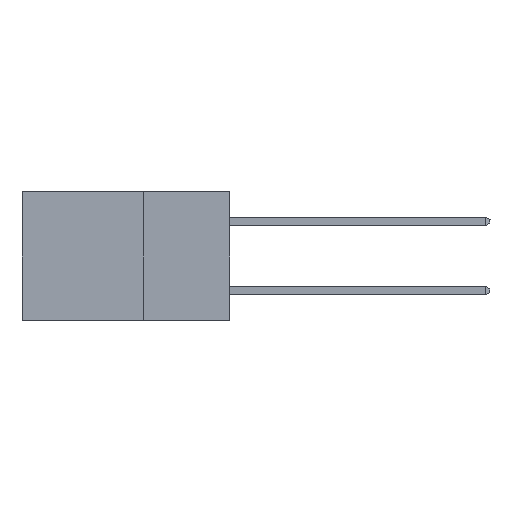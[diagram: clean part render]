
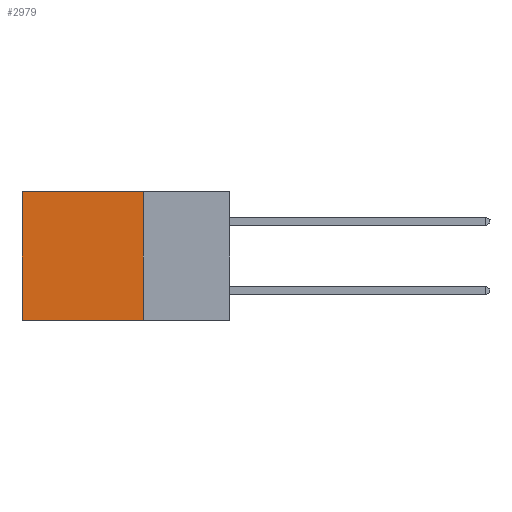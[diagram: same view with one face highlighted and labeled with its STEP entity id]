
A CAD part, left-side view. The second image highlights one B-rep face of the part: STEP entity #2979.
In plain terms, the highlighted planar face has unit normal (-1, 0, 0).
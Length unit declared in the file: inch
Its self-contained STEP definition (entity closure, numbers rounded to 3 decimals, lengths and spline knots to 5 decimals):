
#1040 = DIRECTION ( 'NONE',  ( 1., 0., 0. ) ) ;
#2979 = ADVANCED_FACE ( 'NONE', ( #11093 ), #12424, .F. ) ;
#3132 = AXIS2_PLACEMENT_3D ( 'NONE', #5033, #1040, #6096 ) ;
#3693 = EDGE_CURVE ( 'NONE', #15680, #8187, #13359, .T. ) ;
#4676 = VECTOR ( 'NONE', #14697, 39.37008 ) ;
#4803 = DIRECTION ( 'NONE',  ( 0., 1., 0. ) ) ;
#5033 = CARTESIAN_POINT ( 'NONE',  ( 0.2615, 0.25, -0.37 ) ) ;
#5502 = VECTOR ( 'NONE', #9378, 39.37008 ) ;
#5629 = CARTESIAN_POINT ( 'NONE',  ( 0.2615, 0.25, -0.37 ) ) ;
#6096 = DIRECTION ( 'NONE',  ( 0., 0., -1. ) ) ;
#6901 = EDGE_CURVE ( 'NONE', #7925, #8187, #10790, .T. ) ;
#7024 = CARTESIAN_POINT ( 'NONE',  ( 0.2615, 0.25, -0.37 ) ) ;
#7925 = VERTEX_POINT ( 'NONE', #5629 ) ;
#8187 = VERTEX_POINT ( 'NONE', #14788 ) ;
#9378 = DIRECTION ( 'NONE',  ( 0., 0., -1. ) ) ;
#9554 = LINE ( 'NONE', #15711, #5502 ) ;
#9958 = CARTESIAN_POINT ( 'NONE',  ( 0.2615, 0.25, 0. ) ) ;
#10339 = ORIENTED_EDGE ( 'NONE', *, *, #14576, .F. ) ;
#10790 = LINE ( 'NONE', #7024, #4676 ) ;
#10942 = CARTESIAN_POINT ( 'NONE',  ( 0.2615, 0.6, -0.37 ) ) ;
#11063 = ORIENTED_EDGE ( 'NONE', *, *, #6901, .F. ) ;
#11093 = FACE_OUTER_BOUND ( 'NONE', #15343, .T. ) ;
#11129 = LINE ( 'NONE', #9958, #15327 ) ;
#11889 = CARTESIAN_POINT ( 'NONE',  ( 0.2615, 0.6, 0. ) ) ;
#12424 = PLANE ( 'NONE',  #3132 ) ;
#12486 = ORIENTED_EDGE ( 'NONE', *, *, #14134, .T. ) ;
#12831 = VECTOR ( 'NONE', #16021, 39.37008 ) ;
#13359 = LINE ( 'NONE', #10942, #12831 ) ;
#13715 = VERTEX_POINT ( 'NONE', #15216 ) ;
#14134 = EDGE_CURVE ( 'NONE', #13715, #15680, #11129, .T. ) ;
#14576 = EDGE_CURVE ( 'NONE', #13715, #7925, #9554, .T. ) ;
#14697 = DIRECTION ( 'NONE',  ( 0., 1., 0. ) ) ;
#14788 = CARTESIAN_POINT ( 'NONE',  ( 0.2615, 0.6, -0.37 ) ) ;
#15216 = CARTESIAN_POINT ( 'NONE',  ( 0.2615, 0.25, 0. ) ) ;
#15327 = VECTOR ( 'NONE', #4803, 39.37008 ) ;
#15343 = EDGE_LOOP ( 'NONE', ( #15404, #11063, #10339, #12486 ) ) ;
#15404 = ORIENTED_EDGE ( 'NONE', *, *, #3693, .T. ) ;
#15680 = VERTEX_POINT ( 'NONE', #11889 ) ;
#15711 = CARTESIAN_POINT ( 'NONE',  ( 0.2615, 0.25, -0.37 ) ) ;
#16021 = DIRECTION ( 'NONE',  ( 0., 0., -1. ) ) ;
